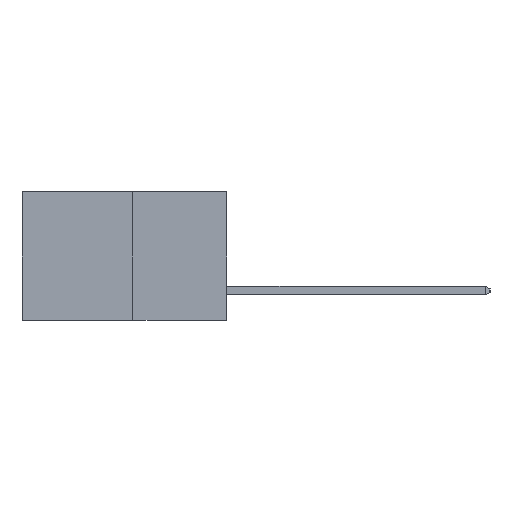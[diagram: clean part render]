
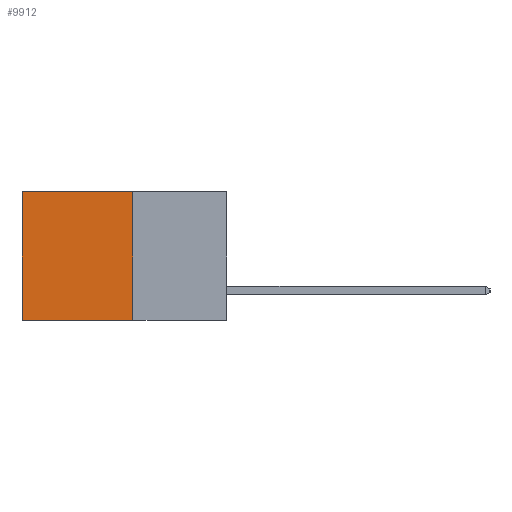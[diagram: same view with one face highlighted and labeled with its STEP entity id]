
A CAD part, left-side view. The second image highlights one B-rep face of the part: STEP entity #9912.
In plain terms, the highlighted planar face has unit normal (-1, 0, 0).
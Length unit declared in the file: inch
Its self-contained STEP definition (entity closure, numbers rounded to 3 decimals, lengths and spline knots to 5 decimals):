
#906 = ORIENTED_EDGE ( 'NONE', *, *, #6219, .T. ) ;
#1380 = LINE ( 'NONE', #12361, #15314 ) ;
#1631 = VECTOR ( 'NONE', #14165, 39.37008 ) ;
#2252 = CARTESIAN_POINT ( 'NONE',  ( 0.277, 0.27, -0.37 ) ) ;
#2936 = LINE ( 'NONE', #6215, #6203 ) ;
#3781 = VERTEX_POINT ( 'NONE', #4975 ) ;
#4207 = CARTESIAN_POINT ( 'NONE',  ( 0.277, 0.27, 0. ) ) ;
#4975 = CARTESIAN_POINT ( 'NONE',  ( 0.277, 0.59, -0.37 ) ) ;
#5547 = EDGE_CURVE ( 'NONE', #11983, #13434, #16374, .T. ) ;
#5833 = CARTESIAN_POINT ( 'NONE',  ( 0.277, 0.27, 0. ) ) ;
#5937 = EDGE_CURVE ( 'NONE', #11983, #17398, #2936, .T. ) ;
#6203 = VECTOR ( 'NONE', #17249, 39.37008 ) ;
#6215 = CARTESIAN_POINT ( 'NONE',  ( 0.277, 0.27, -0.37 ) ) ;
#6219 = EDGE_CURVE ( 'NONE', #13434, #3781, #1380, .T. ) ;
#6244 = EDGE_LOOP ( 'NONE', ( #906, #9641, #16582, #11901 ) ) ;
#6711 = PLANE ( 'NONE',  #8185 ) ;
#8074 = DIRECTION ( 'NONE',  ( 0., 0., -1. ) ) ;
#8185 = AXIS2_PLACEMENT_3D ( 'NONE', #17594, #16373, #8074 ) ;
#8679 = CARTESIAN_POINT ( 'NONE',  ( 0.277, 0.59, 0. ) ) ;
#8802 = VECTOR ( 'NONE', #13411, 39.37008 ) ;
#9641 = ORIENTED_EDGE ( 'NONE', *, *, #13060, .F. ) ;
#9912 = ADVANCED_FACE ( 'NONE', ( #14758 ), #6711, .F. ) ;
#11901 = ORIENTED_EDGE ( 'NONE', *, *, #5547, .T. ) ;
#11983 = VERTEX_POINT ( 'NONE', #4207 ) ;
#12361 = CARTESIAN_POINT ( 'NONE',  ( 0.277, 0.59, -0.37 ) ) ;
#12558 = LINE ( 'NONE', #2252, #8802 ) ;
#13060 = EDGE_CURVE ( 'NONE', #17398, #3781, #12558, .T. ) ;
#13411 = DIRECTION ( 'NONE',  ( 0., 1., 0. ) ) ;
#13434 = VERTEX_POINT ( 'NONE', #8679 ) ;
#13761 = DIRECTION ( 'NONE',  ( 0., 0., -1. ) ) ;
#14165 = DIRECTION ( 'NONE',  ( 0., 1., 0. ) ) ;
#14758 = FACE_OUTER_BOUND ( 'NONE', #6244, .T. ) ;
#15314 = VECTOR ( 'NONE', #13761, 39.37008 ) ;
#16373 = DIRECTION ( 'NONE',  ( 1., 0., 0. ) ) ;
#16374 = LINE ( 'NONE', #5833, #1631 ) ;
#16582 = ORIENTED_EDGE ( 'NONE', *, *, #5937, .F. ) ;
#17249 = DIRECTION ( 'NONE',  ( 0., 0., -1. ) ) ;
#17398 = VERTEX_POINT ( 'NONE', #17871 ) ;
#17594 = CARTESIAN_POINT ( 'NONE',  ( 0.277, 0.27, -0.37 ) ) ;
#17871 = CARTESIAN_POINT ( 'NONE',  ( 0.277, 0.27, -0.37 ) ) ;
